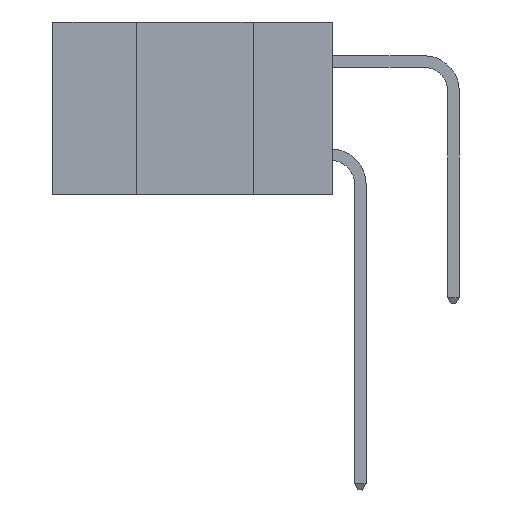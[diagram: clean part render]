
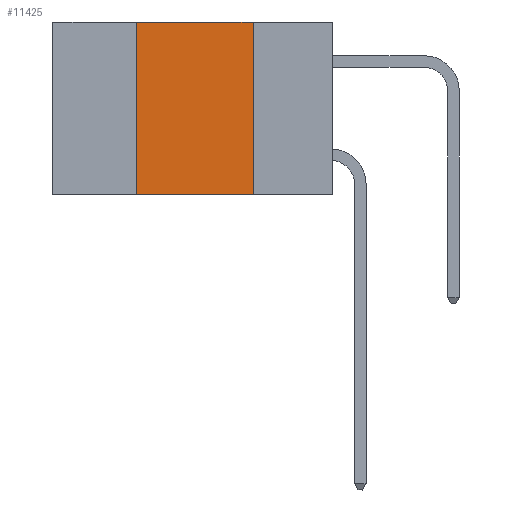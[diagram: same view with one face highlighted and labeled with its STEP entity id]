
A CAD part, left-side view. The second image highlights one B-rep face of the part: STEP entity #11425.
In plain terms, the highlighted planar face has unit normal (-1, 0, 0).
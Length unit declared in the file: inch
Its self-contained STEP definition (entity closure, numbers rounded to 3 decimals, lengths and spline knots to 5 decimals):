
#625 = VECTOR ( 'NONE', #9562, 39.37008 ) ;
#1130 = LINE ( 'NONE', #12672, #625 ) ;
#1756 = CARTESIAN_POINT ( 'NONE',  ( 0., 0.42, 0. ) ) ;
#2014 = ORIENTED_EDGE ( 'NONE', *, *, #14240, .T. ) ;
#2593 = VECTOR ( 'NONE', #18904, 39.37008 ) ;
#3940 = EDGE_LOOP ( 'NONE', ( #16172, #4060, #15222, #2014 ) ) ;
#4060 = ORIENTED_EDGE ( 'NONE', *, *, #5738, .F. ) ;
#4485 = CARTESIAN_POINT ( 'NONE',  ( 0., 0.17, 0. ) ) ;
#5738 = EDGE_CURVE ( 'NONE', #13196, #17224, #5971, .T. ) ;
#5971 = LINE ( 'NONE', #6111, #17707 ) ;
#6111 = CARTESIAN_POINT ( 'NONE',  ( 0., 0.6, 0. ) ) ;
#6116 = DIRECTION ( 'NONE',  ( 0., -1., 0. ) ) ;
#6566 = PLANE ( 'NONE',  #19680 ) ;
#7645 = DIRECTION ( 'NONE',  ( 0., -1., 0. ) ) ;
#8229 = DIRECTION ( 'NONE',  ( 0., 0., -1. ) ) ;
#8650 = FACE_OUTER_BOUND ( 'NONE', #3940, .T. ) ;
#9004 = VERTEX_POINT ( 'NONE', #11677 ) ;
#9562 = DIRECTION ( 'NONE',  ( 0., 0., 1. ) ) ;
#9662 = CARTESIAN_POINT ( 'NONE',  ( 0., 0.17, 0. ) ) ;
#11381 = CARTESIAN_POINT ( 'NONE',  ( 0., 0.6, 0. ) ) ;
#11425 = ADVANCED_FACE ( 'NONE', ( #8650 ), #6566, .F. ) ;
#11677 = CARTESIAN_POINT ( 'NONE',  ( 0., 0.17, -0.37 ) ) ;
#12642 = LINE ( 'NONE', #15617, #16387 ) ;
#12672 = CARTESIAN_POINT ( 'NONE',  ( 0., 0.42, 0. ) ) ;
#12872 = CARTESIAN_POINT ( 'NONE',  ( 0., 0.42, -0.37 ) ) ;
#13196 = VERTEX_POINT ( 'NONE', #1756 ) ;
#14240 = EDGE_CURVE ( 'NONE', #16023, #9004, #12642, .T. ) ;
#15222 = ORIENTED_EDGE ( 'NONE', *, *, #15944, .F. ) ;
#15617 = CARTESIAN_POINT ( 'NONE',  ( 0., 0.6, -0.37 ) ) ;
#15944 = EDGE_CURVE ( 'NONE', #16023, #13196, #1130, .T. ) ;
#16023 = VERTEX_POINT ( 'NONE', #12872 ) ;
#16172 = ORIENTED_EDGE ( 'NONE', *, *, #17076, .F. ) ;
#16387 = VECTOR ( 'NONE', #7645, 39.37008 ) ;
#17076 = EDGE_CURVE ( 'NONE', #17224, #9004, #19227, .T. ) ;
#17224 = VERTEX_POINT ( 'NONE', #9662 ) ;
#17707 = VECTOR ( 'NONE', #6116, 39.37008 ) ;
#17760 = DIRECTION ( 'NONE',  ( 1., 0., 0. ) ) ;
#18904 = DIRECTION ( 'NONE',  ( 0., 0., -1. ) ) ;
#19227 = LINE ( 'NONE', #4485, #2593 ) ;
#19680 = AXIS2_PLACEMENT_3D ( 'NONE', #11381, #17760, #8229 ) ;
